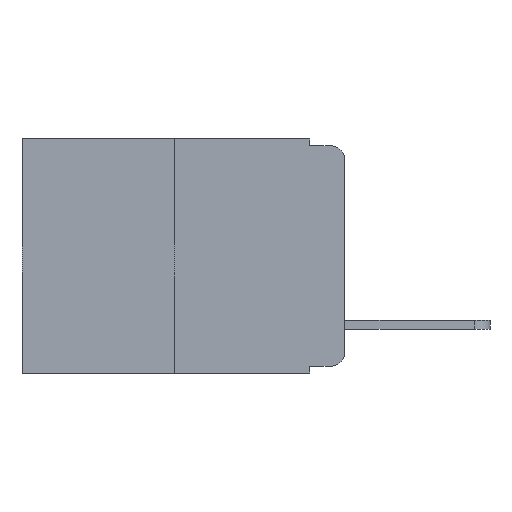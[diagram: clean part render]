
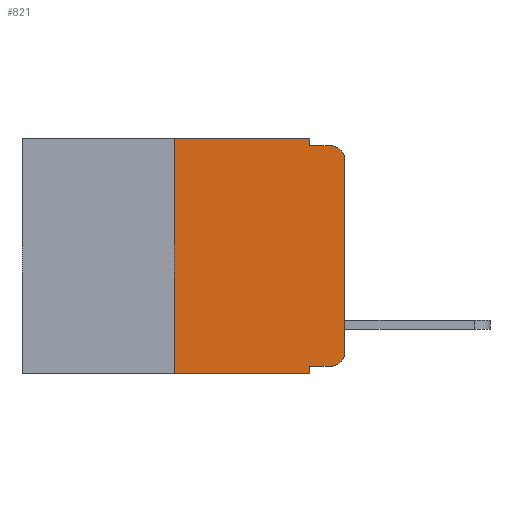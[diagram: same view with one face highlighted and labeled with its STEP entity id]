
A CAD part, left-side view. The second image highlights one B-rep face of the part: STEP entity #821.
In plain terms, the highlighted planar face has unit normal (-1, 0, 0).
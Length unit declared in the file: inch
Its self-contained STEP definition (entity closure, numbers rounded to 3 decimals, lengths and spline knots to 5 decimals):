
#126 = CARTESIAN_POINT ( 'NONE',  ( 0., 0.02, -0.313 ) ) ;
#127 = EDGE_CURVE ( 'NONE', #7277, #17188, #14772, .T. ) ;
#410 = LINE ( 'NONE', #16601, #20185 ) ;
#514 = CARTESIAN_POINT ( 'NONE',  ( 0., 0.051, -0.333 ) ) ;
#692 = VERTEX_POINT ( 'NONE', #14784 ) ;
#821 = ADVANCED_FACE ( 'NONE', ( #12083 ), #8925, .F. ) ;
#827 = EDGE_CURVE ( 'NONE', #11902, #10204, #15814, .T. ) ;
#1602 = EDGE_CURVE ( 'NONE', #17188, #7135, #15569, .T. ) ;
#1820 = CARTESIAN_POINT ( 'NONE',  ( 0., 0.051, 0. ) ) ;
#1840 = VERTEX_POINT ( 'NONE', #14830 ) ;
#2095 = CARTESIAN_POINT ( 'NONE',  ( 0., 0.473, -0.343 ) ) ;
#2617 = CARTESIAN_POINT ( 'NONE',  ( 0., 0., -0.313 ) ) ;
#2925 = VERTEX_POINT ( 'NONE', #20201 ) ;
#2957 = AXIS2_PLACEMENT_3D ( 'NONE', #18308, #8897, #18406 ) ;
#2977 = DIRECTION ( 'NONE',  ( 0., -1., 0. ) ) ;
#3050 = VECTOR ( 'NONE', #19098, 39.37008 ) ;
#3631 = LINE ( 'NONE', #12306, #3050 ) ;
#3708 = VERTEX_POINT ( 'NONE', #12192 ) ;
#3720 = DIRECTION ( 'NONE',  ( 0., 0., -1. ) ) ;
#4154 = ORIENTED_EDGE ( 'NONE', *, *, #1602, .T. ) ;
#4643 = CARTESIAN_POINT ( 'NONE',  ( 0., 0.051, -0.343 ) ) ;
#5770 = ORIENTED_EDGE ( 'NONE', *, *, #7831, .T. ) ;
#5953 = DIRECTION ( 'NONE',  ( 0., 0., -1. ) ) ;
#6570 = VECTOR ( 'NONE', #20301, 39.37008 ) ;
#6732 = VECTOR ( 'NONE', #3720, 39.37008 ) ;
#6826 = EDGE_CURVE ( 'NONE', #3708, #1840, #20017, .T. ) ;
#6928 = DIRECTION ( 'NONE',  ( -1., 0., 0. ) ) ;
#7124 = CARTESIAN_POINT ( 'NONE',  ( 0., 0.051, 0. ) ) ;
#7135 = VERTEX_POINT ( 'NONE', #2617 ) ;
#7173 = LINE ( 'NONE', #8484, #10966 ) ;
#7210 = ORIENTED_EDGE ( 'NONE', *, *, #127, .T. ) ;
#7249 = LINE ( 'NONE', #1820, #6732 ) ;
#7277 = VERTEX_POINT ( 'NONE', #11686 ) ;
#7362 = VECTOR ( 'NONE', #17004, 39.37008 ) ;
#7541 = EDGE_CURVE ( 'NONE', #692, #19631, #410, .T. ) ;
#7831 = EDGE_CURVE ( 'NONE', #7135, #2925, #17274, .T. ) ;
#8484 = CARTESIAN_POINT ( 'NONE',  ( 0., 0.051, 0. ) ) ;
#8583 = EDGE_CURVE ( 'NONE', #7277, #10204, #7249, .T. ) ;
#8706 = ORIENTED_EDGE ( 'NONE', *, *, #16842, .F. ) ;
#8727 = ORIENTED_EDGE ( 'NONE', *, *, #8583, .F. ) ;
#8897 = DIRECTION ( 'NONE',  ( 1., 0., 0. ) ) ;
#8925 = PLANE ( 'NONE',  #2957 ) ;
#9005 = ORIENTED_EDGE ( 'NONE', *, *, #6826, .F. ) ;
#9581 = ORIENTED_EDGE ( 'NONE', *, *, #15679, .T. ) ;
#9630 = VECTOR ( 'NONE', #11977, 39.37008 ) ;
#9918 = DIRECTION ( 'NONE',  ( -1., 0., 0. ) ) ;
#10204 = VERTEX_POINT ( 'NONE', #4643 ) ;
#10377 = CARTESIAN_POINT ( 'NONE',  ( 0., 0., 0. ) ) ;
#10379 = EDGE_CURVE ( 'NONE', #19631, #3708, #7173, .T. ) ;
#10966 = VECTOR ( 'NONE', #14571, 39.37008 ) ;
#11427 = ORIENTED_EDGE ( 'NONE', *, *, #7541, .F. ) ;
#11665 = ORIENTED_EDGE ( 'NONE', *, *, #827, .T. ) ;
#11686 = CARTESIAN_POINT ( 'NONE',  ( 0., 0.051, -0.333 ) ) ;
#11902 = VERTEX_POINT ( 'NONE', #14642 ) ;
#11977 = DIRECTION ( 'NONE',  ( 0., 0., 1. ) ) ;
#12083 = FACE_OUTER_BOUND ( 'NONE', #18211, .T. ) ;
#12156 = ORIENTED_EDGE ( 'NONE', *, *, #10379, .F. ) ;
#12192 = CARTESIAN_POINT ( 'NONE',  ( 0., 0.051, -0.01 ) ) ;
#12306 = CARTESIAN_POINT ( 'NONE',  ( 0., 0.25, 0. ) ) ;
#12731 = AXIS2_PLACEMENT_3D ( 'NONE', #18408, #9918, #19750 ) ;
#12967 = CARTESIAN_POINT ( 'NONE',  ( 0., 0.051, -0.01 ) ) ;
#14571 = DIRECTION ( 'NONE',  ( 0., 0., -1. ) ) ;
#14642 = CARTESIAN_POINT ( 'NONE',  ( 0., 0.25, -0.343 ) ) ;
#14772 = LINE ( 'NONE', #514, #6570 ) ;
#14784 = CARTESIAN_POINT ( 'NONE',  ( 0., 0.25, 0. ) ) ;
#14830 = CARTESIAN_POINT ( 'NONE',  ( 0., 0.02, -0.01 ) ) ;
#15569 = CIRCLE ( 'NONE', #19848, 0.02 ) ;
#15679 = EDGE_CURVE ( 'NONE', #2925, #1840, #16362, .T. ) ;
#15814 = LINE ( 'NONE', #2095, #7362 ) ;
#16362 = CIRCLE ( 'NONE', #12731, 0.02 ) ;
#16449 = VECTOR ( 'NONE', #2977, 39.37008 ) ;
#16601 = CARTESIAN_POINT ( 'NONE',  ( 0., 0.473, 0. ) ) ;
#16662 = DIRECTION ( 'NONE',  ( 0., -1., 0. ) ) ;
#16842 = EDGE_CURVE ( 'NONE', #11902, #692, #3631, .T. ) ;
#17004 = DIRECTION ( 'NONE',  ( 0., -1., 0. ) ) ;
#17188 = VERTEX_POINT ( 'NONE', #19439 ) ;
#17274 = LINE ( 'NONE', #10377, #9630 ) ;
#18211 = EDGE_LOOP ( 'NONE', ( #5770, #9581, #9005, #12156, #11427, #8706, #11665, #8727, #7210, #4154 ) ) ;
#18308 = CARTESIAN_POINT ( 'NONE',  ( 0., 0.473, 0. ) ) ;
#18406 = DIRECTION ( 'NONE',  ( 0., 0., -1. ) ) ;
#18408 = CARTESIAN_POINT ( 'NONE',  ( 0., 0.02, -0.03 ) ) ;
#19098 = DIRECTION ( 'NONE',  ( 0., 0., 1. ) ) ;
#19439 = CARTESIAN_POINT ( 'NONE',  ( 0., 0.02, -0.333 ) ) ;
#19631 = VERTEX_POINT ( 'NONE', #7124 ) ;
#19750 = DIRECTION ( 'NONE',  ( 0., 0., -1. ) ) ;
#19848 = AXIS2_PLACEMENT_3D ( 'NONE', #126, #6928, #5953 ) ;
#20017 = LINE ( 'NONE', #12967, #16449 ) ;
#20185 = VECTOR ( 'NONE', #16662, 39.37008 ) ;
#20201 = CARTESIAN_POINT ( 'NONE',  ( 0., 0., -0.03 ) ) ;
#20301 = DIRECTION ( 'NONE',  ( 0., -1., 0. ) ) ;
